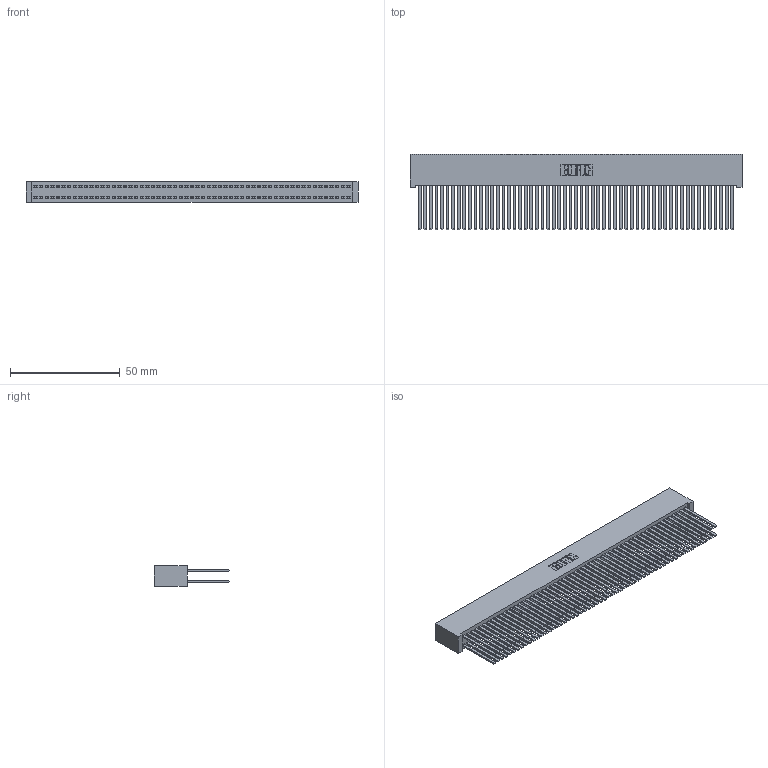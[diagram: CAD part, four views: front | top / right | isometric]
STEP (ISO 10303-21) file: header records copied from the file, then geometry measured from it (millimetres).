
FILE_DESCRIPTION (( 'STEP AP203' ), '1' );
FILE_NAME ('392-114-544-201.STEP', '2019-10-10T01:09:37', ( '' ), ( '' ), 'SwSTEP 2.0', 'SolidWorks 2016', '' );
FILE_SCHEMA (( 'CONFIG_CONTROL_DESIGN' ));
Length unit declared in the file: inch
Products named in the file (3): 342 Part_Lugless; 345-292-001_345-293-144; 392-114-544-201
Assembly tree (115 placements, depth 2):
  392-114-544-201
    342 Part_Lugless
    345-292-001_345-293-144  x114
Bounding box: 151.03 x 34.3 x 9.4 mm (x, y, z)
Volume: 15678.5 mm3; surface area: 30762.1 mm2
Topology: 115 solids, 115 shells, 5346 faces, 15893 edges, 10442 vertices
Faces by surface type: plane 3710, cylinder 1636
Entity records: 34137 total; most frequent: CARTESIAN_POINT 5634, ORIENTED_EDGE 5570, DIRECTION 4777, EDGE_CURVE 2785, VECTOR 2669, LINE 2669, VERTEX_POINT 1854, AXIS2_PLACEMENT_3D 1054
